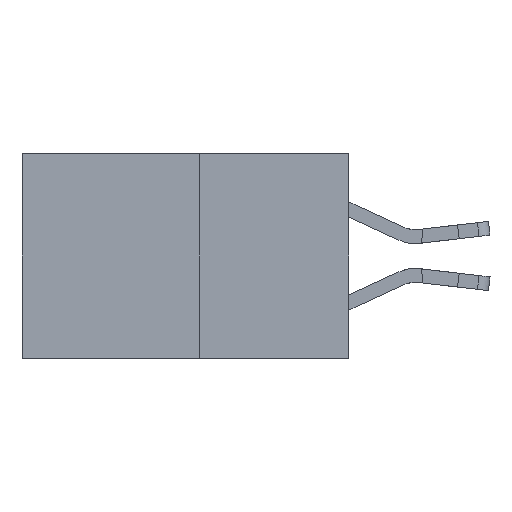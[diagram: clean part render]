
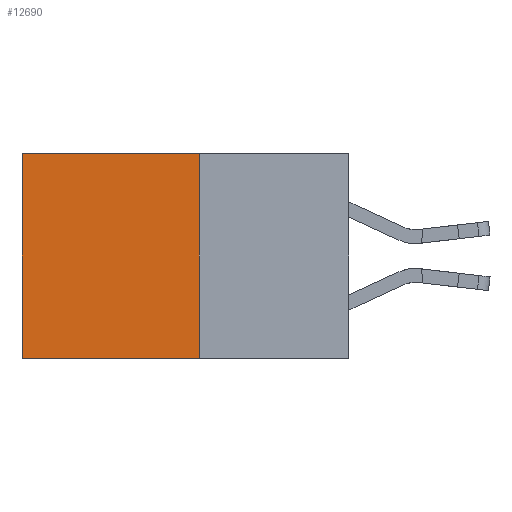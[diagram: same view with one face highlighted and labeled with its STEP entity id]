
A CAD part, left-side view. The second image highlights one B-rep face of the part: STEP entity #12690.
In plain terms, the highlighted planar face has unit normal (-1, 0, 0).
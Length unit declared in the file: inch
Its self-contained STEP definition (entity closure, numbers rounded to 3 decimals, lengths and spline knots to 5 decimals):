
#288 = VECTOR ( 'NONE', #11351, 39.37008 ) ;
#449 = VERTEX_POINT ( 'NONE', #14577 ) ;
#691 = LINE ( 'NONE', #11478, #288 ) ;
#1653 = CARTESIAN_POINT ( 'NONE',  ( 0.277, 0.27, 0. ) ) ;
#2830 = DIRECTION ( 'NONE',  ( 0., 0., -1. ) ) ;
#3559 = DIRECTION ( 'NONE',  ( 0., 0., -1. ) ) ;
#3992 = VERTEX_POINT ( 'NONE', #1653 ) ;
#4736 = ORIENTED_EDGE ( 'NONE', *, *, #6335, .T. ) ;
#4929 = ORIENTED_EDGE ( 'NONE', *, *, #8202, .T. ) ;
#5241 = CARTESIAN_POINT ( 'NONE',  ( 0.277, 0.27, -0.37 ) ) ;
#5779 = DIRECTION ( 'NONE',  ( 0., 0., -1. ) ) ;
#6335 = EDGE_CURVE ( 'NONE', #3992, #449, #691, .T. ) ;
#6529 = ORIENTED_EDGE ( 'NONE', *, *, #9835, .F. ) ;
#7767 = PLANE ( 'NONE',  #15069 ) ;
#8008 = EDGE_LOOP ( 'NONE', ( #4929, #6529, #8173, #4736 ) ) ;
#8173 = ORIENTED_EDGE ( 'NONE', *, *, #10881, .F. ) ;
#8202 = EDGE_CURVE ( 'NONE', #449, #13471, #9224, .T. ) ;
#9000 = CARTESIAN_POINT ( 'NONE',  ( 0.277, 0.27, -0.37 ) ) ;
#9011 = CARTESIAN_POINT ( 'NONE',  ( 0.277, 0.59, -0.37 ) ) ;
#9199 = DIRECTION ( 'NONE',  ( 0., 1., 0. ) ) ;
#9224 = LINE ( 'NONE', #10998, #15785 ) ;
#9588 = VECTOR ( 'NONE', #9199, 39.37008 ) ;
#9835 = EDGE_CURVE ( 'NONE', #13431, #13471, #12894, .T. ) ;
#10259 = DIRECTION ( 'NONE',  ( 1., 0., 0. ) ) ;
#10405 = CARTESIAN_POINT ( 'NONE',  ( 0.277, 0.27, -0.37 ) ) ;
#10881 = EDGE_CURVE ( 'NONE', #3992, #13431, #10934, .T. ) ;
#10934 = LINE ( 'NONE', #13195, #11295 ) ;
#10998 = CARTESIAN_POINT ( 'NONE',  ( 0.277, 0.59, -0.37 ) ) ;
#11239 = FACE_OUTER_BOUND ( 'NONE', #8008, .T. ) ;
#11295 = VECTOR ( 'NONE', #5779, 39.37008 ) ;
#11351 = DIRECTION ( 'NONE',  ( 0., 1., 0. ) ) ;
#11478 = CARTESIAN_POINT ( 'NONE',  ( 0.277, 0.27, 0. ) ) ;
#12690 = ADVANCED_FACE ( 'NONE', ( #11239 ), #7767, .F. ) ;
#12894 = LINE ( 'NONE', #10405, #9588 ) ;
#13195 = CARTESIAN_POINT ( 'NONE',  ( 0.277, 0.27, -0.37 ) ) ;
#13431 = VERTEX_POINT ( 'NONE', #5241 ) ;
#13471 = VERTEX_POINT ( 'NONE', #9011 ) ;
#14577 = CARTESIAN_POINT ( 'NONE',  ( 0.277, 0.59, 0. ) ) ;
#15069 = AXIS2_PLACEMENT_3D ( 'NONE', #9000, #10259, #2830 ) ;
#15785 = VECTOR ( 'NONE', #3559, 39.37008 ) ;
